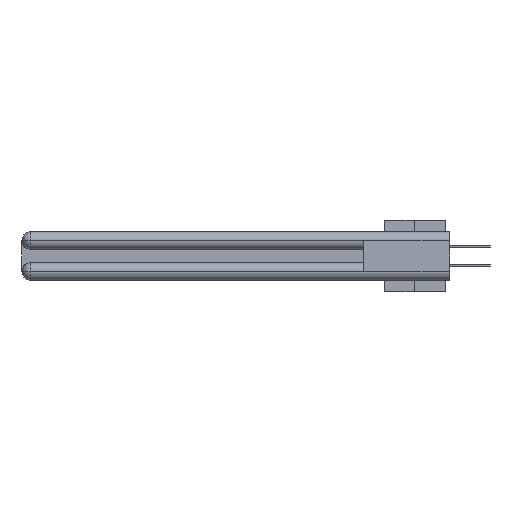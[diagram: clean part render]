
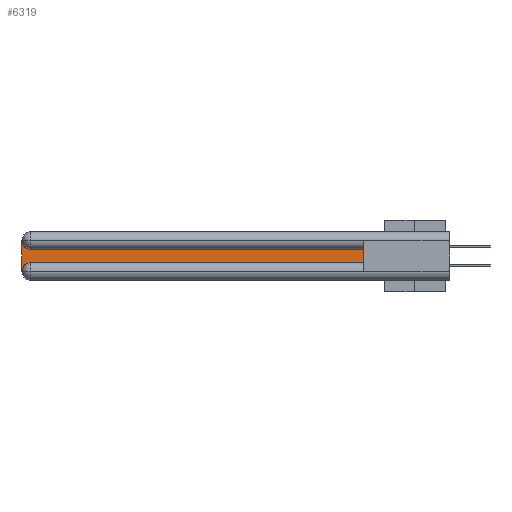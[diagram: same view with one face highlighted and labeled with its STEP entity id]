
A CAD part, left-side view. The second image highlights one B-rep face of the part: STEP entity #6319.
In plain terms, the highlighted planar face has unit normal (-1, 0, 0).
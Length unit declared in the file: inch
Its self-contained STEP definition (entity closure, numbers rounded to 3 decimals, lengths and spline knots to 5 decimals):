
#1425 = LINE ( 'NONE', #11393, #11981 ) ;
#2110 = LINE ( 'NONE', #25165, #41699 ) ;
#2193 = FACE_OUTER_BOUND ( 'NONE', #10323, .T. ) ;
#2442 = CARTESIAN_POINT ( 'NONE',  ( 0.075, 2.94, -0.2175 ) ) ;
#3402 = CIRCLE ( 'NONE', #25429, 0.06 ) ;
#4723 = EDGE_CURVE ( 'NONE', #19003, #44883, #30245, .T. ) ;
#5032 = CARTESIAN_POINT ( 'NONE',  ( 0.075, 0.6, -0.1225 ) ) ;
#5937 = CARTESIAN_POINT ( 'NONE',  ( 0.075, 0.6, -0.2175 ) ) ;
#6319 = ADVANCED_FACE ( 'NONE', ( #2193 ), #12540, .F. ) ;
#9621 = VECTOR ( 'NONE', #18822, 39.37008 ) ;
#10323 = EDGE_LOOP ( 'NONE', ( #22601, #32426, #41829, #41868, #17236, #35316 ) ) ;
#11393 = CARTESIAN_POINT ( 'NONE',  ( 0.075, 0.6, -0.1225 ) ) ;
#11981 = VECTOR ( 'NONE', #29673, 39.37008 ) ;
#12540 = PLANE ( 'NONE',  #24935 ) ;
#12999 = DIRECTION ( 'NONE',  ( 1., 0., 0. ) ) ;
#14856 = CIRCLE ( 'NONE', #37636, 0.06 ) ;
#15269 = CARTESIAN_POINT ( 'NONE',  ( 0.075, 0.6, -0.2175 ) ) ;
#16330 = CARTESIAN_POINT ( 'NONE',  ( 0.075, 2.94, -0.0625 ) ) ;
#16740 = EDGE_CURVE ( 'NONE', #44848, #17329, #14856, .T. ) ;
#17236 = ORIENTED_EDGE ( 'NONE', *, *, #20770, .T. ) ;
#17329 = VERTEX_POINT ( 'NONE', #2442 ) ;
#17710 = DIRECTION ( 'NONE',  ( 0., 0., -1. ) ) ;
#18822 = DIRECTION ( 'NONE',  ( 0., -1., 0. ) ) ;
#19003 = VERTEX_POINT ( 'NONE', #5937 ) ;
#19582 = EDGE_CURVE ( 'NONE', #27081, #32718, #3402, .T. ) ;
#20770 = EDGE_CURVE ( 'NONE', #17329, #19003, #38614, .T. ) ;
#21688 = CARTESIAN_POINT ( 'NONE',  ( 0.075, 3., -0.0625 ) ) ;
#22601 = ORIENTED_EDGE ( 'NONE', *, *, #31999, .T. ) ;
#23618 = CARTESIAN_POINT ( 'NONE',  ( 0.075, 0.6, -0.2175 ) ) ;
#24935 = AXIS2_PLACEMENT_3D ( 'NONE', #37832, #12999, #37510 ) ;
#25165 = CARTESIAN_POINT ( 'NONE',  ( 0.075, 3., -0.2175 ) ) ;
#25186 = CARTESIAN_POINT ( 'NONE',  ( 0.075, 2.94, -0.2775 ) ) ;
#25429 = AXIS2_PLACEMENT_3D ( 'NONE', #16330, #27077, #41299 ) ;
#27077 = DIRECTION ( 'NONE',  ( 1., 0., 0. ) ) ;
#27081 = VERTEX_POINT ( 'NONE', #43786 ) ;
#29673 = DIRECTION ( 'NONE',  ( 0., 1., 0. ) ) ;
#30245 = LINE ( 'NONE', #23618, #44735 ) ;
#31210 = EDGE_CURVE ( 'NONE', #32718, #44848, #2110, .T. ) ;
#31438 = DIRECTION ( 'NONE',  ( 0., 0., 1. ) ) ;
#31613 = DIRECTION ( 'NONE',  ( 0., 0., -1. ) ) ;
#31999 = EDGE_CURVE ( 'NONE', #44883, #27081, #1425, .T. ) ;
#32426 = ORIENTED_EDGE ( 'NONE', *, *, #19582, .T. ) ;
#32545 = DIRECTION ( 'NONE',  ( 1., 0., 0. ) ) ;
#32718 = VERTEX_POINT ( 'NONE', #21688 ) ;
#35316 = ORIENTED_EDGE ( 'NONE', *, *, #4723, .T. ) ;
#36874 = CARTESIAN_POINT ( 'NONE',  ( 0.075, 3., -0.2775 ) ) ;
#37510 = DIRECTION ( 'NONE',  ( 0., 0., -1. ) ) ;
#37636 = AXIS2_PLACEMENT_3D ( 'NONE', #25186, #32545, #17710 ) ;
#37832 = CARTESIAN_POINT ( 'NONE',  ( 0.075, 3., -0.1225 ) ) ;
#38614 = LINE ( 'NONE', #15269, #9621 ) ;
#41299 = DIRECTION ( 'NONE',  ( 0., 0., -1. ) ) ;
#41699 = VECTOR ( 'NONE', #31613, 39.37008 ) ;
#41829 = ORIENTED_EDGE ( 'NONE', *, *, #31210, .T. ) ;
#41868 = ORIENTED_EDGE ( 'NONE', *, *, #16740, .T. ) ;
#43786 = CARTESIAN_POINT ( 'NONE',  ( 0.075, 2.94, -0.1225 ) ) ;
#44735 = VECTOR ( 'NONE', #31438, 39.37008 ) ;
#44848 = VERTEX_POINT ( 'NONE', #36874 ) ;
#44883 = VERTEX_POINT ( 'NONE', #5032 ) ;
